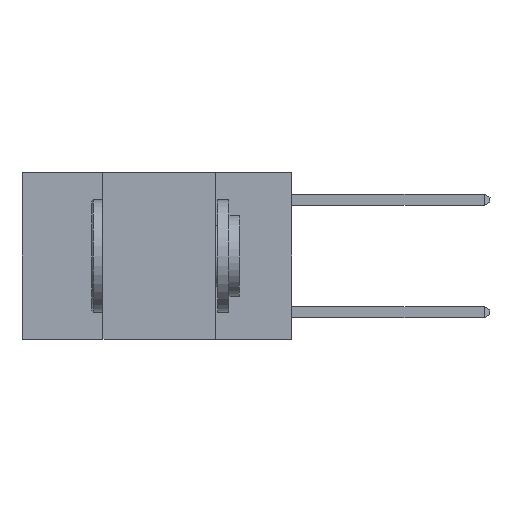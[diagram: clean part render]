
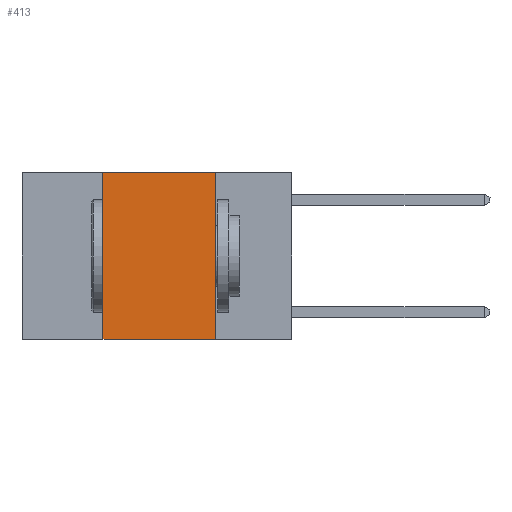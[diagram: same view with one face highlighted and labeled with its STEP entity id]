
A CAD part, left-side view. The second image highlights one B-rep face of the part: STEP entity #413.
In plain terms, the highlighted planar face has unit normal (-1, 0, 0).
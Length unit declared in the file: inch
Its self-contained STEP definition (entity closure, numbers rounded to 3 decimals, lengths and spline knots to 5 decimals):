
#125 = FACE_OUTER_BOUND ( 'NONE', #6030, .T. ) ;
#144 = ORIENTED_EDGE ( 'NONE', *, *, #838, .F. ) ;
#308 = VERTEX_POINT ( 'NONE', #2202 ) ;
#413 = ADVANCED_FACE ( 'NONE', ( #125 ), #6308, .F. ) ;
#838 = EDGE_CURVE ( 'NONE', #6186, #4678, #6319, .T. ) ;
#982 = DIRECTION ( 'NONE',  ( 0., -1., 0. ) ) ;
#1804 = EDGE_CURVE ( 'NONE', #3331, #6186, #5688, .T. ) ;
#1905 = CARTESIAN_POINT ( 'NONE',  ( 0., 0.42, 0. ) ) ;
#2140 = LINE ( 'NONE', #5741, #7215 ) ;
#2146 = ORIENTED_EDGE ( 'NONE', *, *, #8620, .F. ) ;
#2158 = VECTOR ( 'NONE', #7335, 39.37008 ) ;
#2202 = CARTESIAN_POINT ( 'NONE',  ( 0., 0.17, -0.37 ) ) ;
#2273 = EDGE_CURVE ( 'NONE', #3331, #308, #5478, .T. ) ;
#2475 = CARTESIAN_POINT ( 'NONE',  ( 0., 0.6, 0. ) ) ;
#2561 = ORIENTED_EDGE ( 'NONE', *, *, #1804, .F. ) ;
#3108 = CARTESIAN_POINT ( 'NONE',  ( 0., 0.17, 0. ) ) ;
#3331 = VERTEX_POINT ( 'NONE', #7349 ) ;
#4478 = VECTOR ( 'NONE', #5732, 39.37008 ) ;
#4638 = DIRECTION ( 'NONE',  ( 0., 0., -1. ) ) ;
#4678 = VERTEX_POINT ( 'NONE', #3108 ) ;
#5207 = AXIS2_PLACEMENT_3D ( 'NONE', #2475, #5378, #4638 ) ;
#5378 = DIRECTION ( 'NONE',  ( 1., 0., 0. ) ) ;
#5478 = LINE ( 'NONE', #8398, #8671 ) ;
#5650 = DIRECTION ( 'NONE',  ( 0., 0., -1. ) ) ;
#5688 = LINE ( 'NONE', #1905, #4478 ) ;
#5732 = DIRECTION ( 'NONE',  ( 0., 0., 1. ) ) ;
#5741 = CARTESIAN_POINT ( 'NONE',  ( 0., 0.17, 0. ) ) ;
#5961 = CARTESIAN_POINT ( 'NONE',  ( 0., 0.42, 0. ) ) ;
#6030 = EDGE_LOOP ( 'NONE', ( #2146, #144, #2561, #7691 ) ) ;
#6186 = VERTEX_POINT ( 'NONE', #5961 ) ;
#6308 = PLANE ( 'NONE',  #5207 ) ;
#6319 = LINE ( 'NONE', #9246, #2158 ) ;
#7215 = VECTOR ( 'NONE', #5650, 39.37008 ) ;
#7335 = DIRECTION ( 'NONE',  ( 0., -1., 0. ) ) ;
#7349 = CARTESIAN_POINT ( 'NONE',  ( 0., 0.42, -0.37 ) ) ;
#7691 = ORIENTED_EDGE ( 'NONE', *, *, #2273, .T. ) ;
#8398 = CARTESIAN_POINT ( 'NONE',  ( 0., 0.6, -0.37 ) ) ;
#8620 = EDGE_CURVE ( 'NONE', #4678, #308, #2140, .T. ) ;
#8671 = VECTOR ( 'NONE', #982, 39.37008 ) ;
#9246 = CARTESIAN_POINT ( 'NONE',  ( 0., 0.6, 0. ) ) ;
